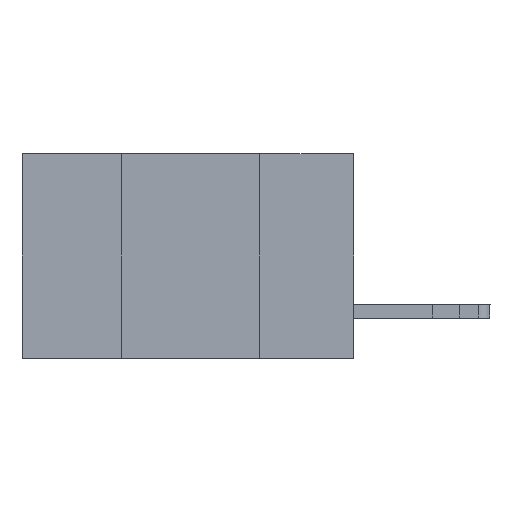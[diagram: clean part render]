
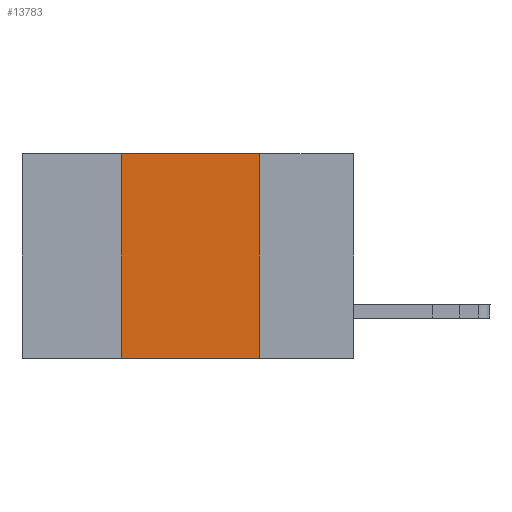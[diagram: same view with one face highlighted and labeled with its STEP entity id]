
A CAD part, left-side view. The second image highlights one B-rep face of the part: STEP entity #13783.
In plain terms, the highlighted planar face has unit normal (-1, 0, 0).
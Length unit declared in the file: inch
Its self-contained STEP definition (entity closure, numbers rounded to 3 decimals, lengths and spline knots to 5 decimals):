
#910 = VERTEX_POINT ( 'NONE', #7098 ) ;
#929 = FACE_OUTER_BOUND ( 'NONE', #8523, .T. ) ;
#1198 = DIRECTION ( 'NONE',  ( 0., 0., -1. ) ) ;
#1547 = DIRECTION ( 'NONE',  ( 0., 0., 1. ) ) ;
#2400 = PLANE ( 'NONE',  #10010 ) ;
#2564 = VERTEX_POINT ( 'NONE', #6095 ) ;
#2796 = DIRECTION ( 'NONE',  ( 1., 0., 0. ) ) ;
#3456 = VERTEX_POINT ( 'NONE', #18167 ) ;
#5306 = DIRECTION ( 'NONE',  ( 0., -1., 0. ) ) ;
#5847 = EDGE_CURVE ( 'NONE', #3456, #910, #17549, .T. ) ;
#6095 = CARTESIAN_POINT ( 'NONE',  ( 0., 0.17, 0. ) ) ;
#6640 = EDGE_CURVE ( 'NONE', #2564, #910, #11071, .T. ) ;
#7098 = CARTESIAN_POINT ( 'NONE',  ( 0., 0.17, -0.37 ) ) ;
#7663 = LINE ( 'NONE', #15699, #13289 ) ;
#7865 = ORIENTED_EDGE ( 'NONE', *, *, #7942, .F. ) ;
#7942 = EDGE_CURVE ( 'NONE', #3456, #15727, #7663, .T. ) ;
#8148 = ORIENTED_EDGE ( 'NONE', *, *, #6640, .F. ) ;
#8523 = EDGE_LOOP ( 'NONE', ( #8148, #13708, #7865, #12511 ) ) ;
#10010 = AXIS2_PLACEMENT_3D ( 'NONE', #16976, #2796, #1198 ) ;
#10971 = CARTESIAN_POINT ( 'NONE',  ( 0., 0.17, 0. ) ) ;
#11071 = LINE ( 'NONE', #10971, #18310 ) ;
#11404 = CARTESIAN_POINT ( 'NONE',  ( 0., 0.6, -0.37 ) ) ;
#12453 = LINE ( 'NONE', #13808, #14467 ) ;
#12495 = EDGE_CURVE ( 'NONE', #15727, #2564, #12453, .T. ) ;
#12511 = ORIENTED_EDGE ( 'NONE', *, *, #5847, .T. ) ;
#13289 = VECTOR ( 'NONE', #1547, 39.37008 ) ;
#13682 = VECTOR ( 'NONE', #18548, 39.37008 ) ;
#13708 = ORIENTED_EDGE ( 'NONE', *, *, #12495, .F. ) ;
#13783 = ADVANCED_FACE ( 'NONE', ( #929 ), #2400, .F. ) ;
#13808 = CARTESIAN_POINT ( 'NONE',  ( 0., 0.6, 0. ) ) ;
#14467 = VECTOR ( 'NONE', #5306, 39.37008 ) ;
#15699 = CARTESIAN_POINT ( 'NONE',  ( 0., 0.42, 0. ) ) ;
#15727 = VERTEX_POINT ( 'NONE', #18334 ) ;
#16976 = CARTESIAN_POINT ( 'NONE',  ( 0., 0.6, 0. ) ) ;
#17178 = DIRECTION ( 'NONE',  ( 0., 0., -1. ) ) ;
#17549 = LINE ( 'NONE', #11404, #13682 ) ;
#18167 = CARTESIAN_POINT ( 'NONE',  ( 0., 0.42, -0.37 ) ) ;
#18310 = VECTOR ( 'NONE', #17178, 39.37008 ) ;
#18334 = CARTESIAN_POINT ( 'NONE',  ( 0., 0.42, 0. ) ) ;
#18548 = DIRECTION ( 'NONE',  ( 0., -1., 0. ) ) ;
